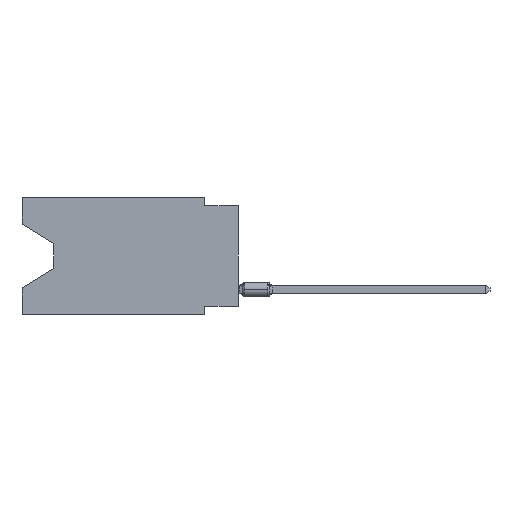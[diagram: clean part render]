
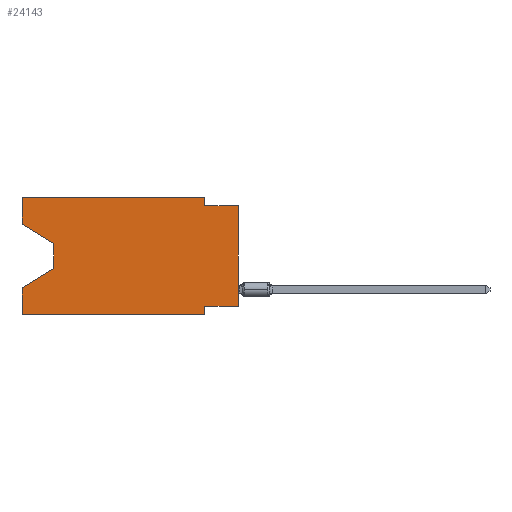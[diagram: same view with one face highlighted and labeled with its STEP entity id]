
A CAD part, left-side view. The second image highlights one B-rep face of the part: STEP entity #24143.
In plain terms, the highlighted planar face has unit normal (-1, 0, 0).
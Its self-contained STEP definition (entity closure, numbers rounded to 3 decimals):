
#626 = DIRECTION ( 'NONE',  ( 0., 1., 0. ) ) ;
#843 = CARTESIAN_POINT ( 'NONE',  ( 0., 13.97, -3.505 ) ) ;
#1133 = ORIENTED_EDGE ( 'NONE', *, *, #14342, .F. ) ;
#1765 = VECTOR ( 'NONE', #20134, 1000. ) ;
#2318 = CARTESIAN_POINT ( 'NONE',  ( 0., 0., -8.255 ) ) ;
#2390 = DIRECTION ( 'NONE',  ( 0., -0.855, -0.519 ) ) ;
#2513 = EDGE_CURVE ( 'NONE', #14080, #19176, #11321, .T. ) ;
#2871 = VECTOR ( 'NONE', #15694, 1000. ) ;
#2939 = CARTESIAN_POINT ( 'NONE',  ( 0., 2.54, -0.635 ) ) ;
#3121 = DIRECTION ( 'NONE',  ( 0., 0., -1. ) ) ;
#3241 = DIRECTION ( 'NONE',  ( 0., 0., -1. ) ) ;
#3801 = ORIENTED_EDGE ( 'NONE', *, *, #27124, .T. ) ;
#4160 = VECTOR ( 'NONE', #11423, 1000. ) ;
#5231 = FACE_OUTER_BOUND ( 'NONE', #12222, .T. ) ;
#5313 = CARTESIAN_POINT ( 'NONE',  ( 0., 0., -8.255 ) ) ;
#5347 = CARTESIAN_POINT ( 'NONE',  ( 0., 16.383, -8.89 ) ) ;
#5432 = EDGE_CURVE ( 'NONE', #15821, #9031, #18101, .T. ) ;
#5488 = ORIENTED_EDGE ( 'NONE', *, *, #15045, .F. ) ;
#5664 = CARTESIAN_POINT ( 'NONE',  ( 0., 2.54, -8.89 ) ) ;
#5701 = DIRECTION ( 'NONE',  ( 1., 0., 0. ) ) ;
#6117 = ORIENTED_EDGE ( 'NONE', *, *, #11902, .T. ) ;
#6165 = CARTESIAN_POINT ( 'NONE',  ( 0., 16.383, 0. ) ) ;
#7062 = DIRECTION ( 'NONE',  ( 0., 0., -1. ) ) ;
#7409 = EDGE_CURVE ( 'NONE', #16182, #17306, #18152, .T. ) ;
#7480 = EDGE_CURVE ( 'NONE', #22077, #14080, #20419, .T. ) ;
#7766 = CARTESIAN_POINT ( 'NONE',  ( 0., 13.97, -3.505 ) ) ;
#8273 = DIRECTION ( 'NONE',  ( 0., 0.855, -0.519 ) ) ;
#8327 = VERTEX_POINT ( 'NONE', #2318 ) ;
#8391 = CARTESIAN_POINT ( 'NONE',  ( 0., 16.383, 0. ) ) ;
#8911 = DIRECTION ( 'NONE',  ( 0., -1., 0. ) ) ;
#9016 = CARTESIAN_POINT ( 'NONE',  ( 0., 16.383, -8.89 ) ) ;
#9031 = VERTEX_POINT ( 'NONE', #15014 ) ;
#9349 = CARTESIAN_POINT ( 'NONE',  ( 0., 16.383, -2.038 ) ) ;
#10036 = VECTOR ( 'NONE', #8273, 1000. ) ;
#10225 = CARTESIAN_POINT ( 'NONE',  ( 0., 0., -0.635 ) ) ;
#10374 = EDGE_CURVE ( 'NONE', #13960, #9031, #17238, .T. ) ;
#10824 = CARTESIAN_POINT ( 'NONE',  ( 0., 2.54, 0. ) ) ;
#11321 = LINE ( 'NONE', #14039, #21281 ) ;
#11423 = DIRECTION ( 'NONE',  ( 0., -1., 0. ) ) ;
#11604 = EDGE_CURVE ( 'NONE', #20771, #27090, #16359, .T. ) ;
#11617 = ORIENTED_EDGE ( 'NONE', *, *, #7480, .F. ) ;
#11902 = EDGE_CURVE ( 'NONE', #8327, #21309, #26996, .T. ) ;
#12222 = EDGE_LOOP ( 'NONE', ( #25771, #3801, #23257, #21045, #21820, #27520, #1133, #6117, #5488, #21221, #11617, #26870 ) ) ;
#12324 = LINE ( 'NONE', #7766, #13177 ) ;
#13177 = VECTOR ( 'NONE', #3241, 1000. ) ;
#13196 = CARTESIAN_POINT ( 'NONE',  ( 0., 13.97, -5.385 ) ) ;
#13273 = CARTESIAN_POINT ( 'NONE',  ( 0., 13.97, -5.385 ) ) ;
#13510 = DIRECTION ( 'NONE',  ( 0., 0., -1. ) ) ;
#13960 = VERTEX_POINT ( 'NONE', #5347 ) ;
#14039 = CARTESIAN_POINT ( 'NONE',  ( 0., 2.54, 0. ) ) ;
#14080 = VERTEX_POINT ( 'NONE', #10824 ) ;
#14342 = EDGE_CURVE ( 'NONE', #8327, #20771, #18944, .T. ) ;
#15014 = CARTESIAN_POINT ( 'NONE',  ( 0., 16.383, -6.852 ) ) ;
#15045 = EDGE_CURVE ( 'NONE', #19176, #21309, #20652, .T. ) ;
#15694 = DIRECTION ( 'NONE',  ( 0., -1., 0. ) ) ;
#15821 = VERTEX_POINT ( 'NONE', #13196 ) ;
#16170 = CARTESIAN_POINT ( 'NONE',  ( 0., 16.383, 0. ) ) ;
#16182 = VERTEX_POINT ( 'NONE', #19821 ) ;
#16201 = CARTESIAN_POINT ( 'NONE',  ( 0., 2.54, -8.89 ) ) ;
#16359 = LINE ( 'NONE', #16201, #23986 ) ;
#17217 = PLANE ( 'NONE',  #19076 ) ;
#17238 = LINE ( 'NONE', #6165, #19901 ) ;
#17306 = VERTEX_POINT ( 'NONE', #843 ) ;
#17425 = EDGE_CURVE ( 'NONE', #16182, #22077, #19912, .T. ) ;
#17688 = CARTESIAN_POINT ( 'NONE',  ( 0., 16.383, 0. ) ) ;
#18101 = LINE ( 'NONE', #13273, #10036 ) ;
#18152 = LINE ( 'NONE', #9349, #21078 ) ;
#18944 = LINE ( 'NONE', #5313, #23006 ) ;
#19076 = AXIS2_PLACEMENT_3D ( 'NONE', #26487, #5701, #3121 ) ;
#19176 = VERTEX_POINT ( 'NONE', #2939 ) ;
#19455 = DIRECTION ( 'NONE',  ( 0., 0., 1. ) ) ;
#19821 = CARTESIAN_POINT ( 'NONE',  ( 0., 16.383, -2.038 ) ) ;
#19901 = VECTOR ( 'NONE', #26503, 1000. ) ;
#19912 = LINE ( 'NONE', #8391, #25902 ) ;
#20134 = DIRECTION ( 'NONE',  ( 0., 0., 1. ) ) ;
#20419 = LINE ( 'NONE', #16170, #22114 ) ;
#20652 = LINE ( 'NONE', #29656, #4160 ) ;
#20771 = VERTEX_POINT ( 'NONE', #23893 ) ;
#21025 = EDGE_CURVE ( 'NONE', #13960, #27090, #27672, .T. ) ;
#21045 = ORIENTED_EDGE ( 'NONE', *, *, #10374, .F. ) ;
#21078 = VECTOR ( 'NONE', #2390, 1000. ) ;
#21221 = ORIENTED_EDGE ( 'NONE', *, *, #2513, .F. ) ;
#21281 = VECTOR ( 'NONE', #7062, 1000. ) ;
#21309 = VERTEX_POINT ( 'NONE', #10225 ) ;
#21820 = ORIENTED_EDGE ( 'NONE', *, *, #21025, .T. ) ;
#22077 = VERTEX_POINT ( 'NONE', #17688 ) ;
#22114 = VECTOR ( 'NONE', #8911, 1000. ) ;
#23006 = VECTOR ( 'NONE', #626, 1000. ) ;
#23257 = ORIENTED_EDGE ( 'NONE', *, *, #5432, .T. ) ;
#23893 = CARTESIAN_POINT ( 'NONE',  ( 0., 2.54, -8.255 ) ) ;
#23986 = VECTOR ( 'NONE', #13510, 1000. ) ;
#24143 = ADVANCED_FACE ( 'NONE', ( #5231 ), #17217, .F. ) ;
#25771 = ORIENTED_EDGE ( 'NONE', *, *, #7409, .T. ) ;
#25902 = VECTOR ( 'NONE', #19455, 1000. ) ;
#26487 = CARTESIAN_POINT ( 'NONE',  ( 0., 16.383, 0. ) ) ;
#26503 = DIRECTION ( 'NONE',  ( 0., 0., 1. ) ) ;
#26870 = ORIENTED_EDGE ( 'NONE', *, *, #17425, .F. ) ;
#26996 = LINE ( 'NONE', #27134, #1765 ) ;
#27090 = VERTEX_POINT ( 'NONE', #5664 ) ;
#27124 = EDGE_CURVE ( 'NONE', #17306, #15821, #12324, .T. ) ;
#27134 = CARTESIAN_POINT ( 'NONE',  ( 0., 0., 0. ) ) ;
#27520 = ORIENTED_EDGE ( 'NONE', *, *, #11604, .F. ) ;
#27672 = LINE ( 'NONE', #9016, #2871 ) ;
#29656 = CARTESIAN_POINT ( 'NONE',  ( 0., 0., -0.635 ) ) ;
